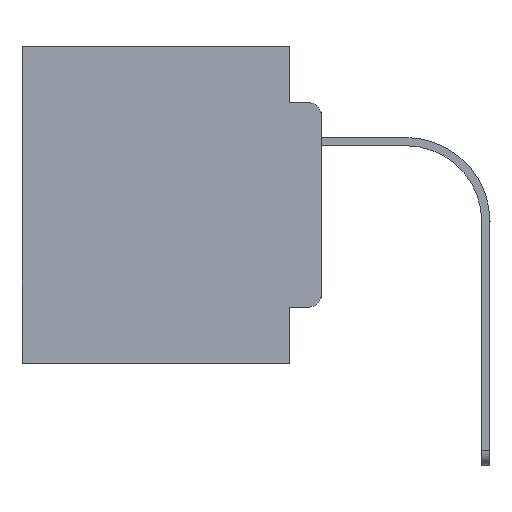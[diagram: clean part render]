
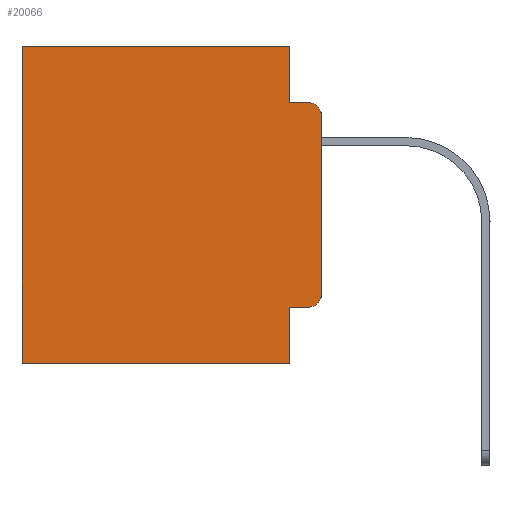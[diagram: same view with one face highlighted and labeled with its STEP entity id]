
A CAD part, left-side view. The second image highlights one B-rep face of the part: STEP entity #20066.
In plain terms, the highlighted planar face has unit normal (-1, 0, 0).
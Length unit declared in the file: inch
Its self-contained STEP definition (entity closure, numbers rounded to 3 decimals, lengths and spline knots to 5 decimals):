
#27 = LINE ( 'NONE', #24233, #23879 ) ;
#28 = DIRECTION ( 'NONE',  ( -1., 0., 0. ) ) ;
#840 = CARTESIAN_POINT ( 'NONE',  ( 0.298, 0.473, 0. ) ) ;
#1230 = ORIENTED_EDGE ( 'NONE', *, *, #2254, .F. ) ;
#1578 = CIRCLE ( 'NONE', #19807, 0.02 ) ;
#1582 = VECTOR ( 'NONE', #14883, 39.37008 ) ;
#1724 = FACE_OUTER_BOUND ( 'NONE', #25973, .T. ) ;
#2254 = EDGE_CURVE ( 'NONE', #10997, #7999, #5723, .T. ) ;
#2486 = EDGE_CURVE ( 'NONE', #16916, #17558, #19081, .T. ) ;
#2746 = CARTESIAN_POINT ( 'NONE',  ( 0.298, 0.02, -0.4115 ) ) ;
#3034 = DIRECTION ( 'NONE',  ( 0., 0., -1. ) ) ;
#3601 = DIRECTION ( 'NONE',  ( 0., 0., -1. ) ) ;
#3669 = EDGE_CURVE ( 'NONE', #10997, #20753, #16736, .T. ) ;
#3742 = CIRCLE ( 'NONE', #19013, 0.02 ) ;
#4521 = CARTESIAN_POINT ( 'NONE',  ( 0.298, 0.051, -0.4115 ) ) ;
#5129 = CARTESIAN_POINT ( 'NONE',  ( 0.298, 0.051, -0.0885 ) ) ;
#5399 = EDGE_CURVE ( 'NONE', #7165, #24015, #1578, .T. ) ;
#5652 = ORIENTED_EDGE ( 'NONE', *, *, #21985, .F. ) ;
#5718 = LINE ( 'NONE', #13822, #18164 ) ;
#5723 = LINE ( 'NONE', #19667, #22315 ) ;
#5754 = EDGE_CURVE ( 'NONE', #20785, #24015, #22165, .T. ) ;
#6103 = EDGE_CURVE ( 'NONE', #20753, #25151, #3742, .T. ) ;
#7036 = ORIENTED_EDGE ( 'NONE', *, *, #2486, .T. ) ;
#7165 = VERTEX_POINT ( 'NONE', #18683 ) ;
#7427 = ORIENTED_EDGE ( 'NONE', *, *, #5754, .F. ) ;
#7999 = VERTEX_POINT ( 'NONE', #25230 ) ;
#8914 = ORIENTED_EDGE ( 'NONE', *, *, #10478, .F. ) ;
#9082 = DIRECTION ( 'NONE',  ( 0., 1., 0. ) ) ;
#9113 = CARTESIAN_POINT ( 'NONE',  ( 0.298, 0., -0.3915 ) ) ;
#9138 = DIRECTION ( 'NONE',  ( 0., 0., -1. ) ) ;
#9844 = DIRECTION ( 'NONE',  ( 0., 1., 0. ) ) ;
#10046 = ORIENTED_EDGE ( 'NONE', *, *, #5399, .T. ) ;
#10109 = CARTESIAN_POINT ( 'NONE',  ( 0.298, 0., 0. ) ) ;
#10478 = EDGE_CURVE ( 'NONE', #7165, #25151, #27, .T. ) ;
#10844 = EDGE_CURVE ( 'NONE', #7999, #17558, #5718, .T. ) ;
#10997 = VERTEX_POINT ( 'NONE', #16455 ) ;
#11525 = DIRECTION ( 'NONE',  ( 0., 0., -1. ) ) ;
#12053 = EDGE_CURVE ( 'NONE', #13106, #16916, #17548, .T. ) ;
#12131 = DIRECTION ( 'NONE',  ( 0., 0., -1. ) ) ;
#12497 = DIRECTION ( 'NONE',  ( 0., 0., -1. ) ) ;
#13106 = VERTEX_POINT ( 'NONE', #16250 ) ;
#13734 = ORIENTED_EDGE ( 'NONE', *, *, #12053, .T. ) ;
#13822 = CARTESIAN_POINT ( 'NONE',  ( 0.298, 0., -0.5 ) ) ;
#14144 = VECTOR ( 'NONE', #9138, 39.37008 ) ;
#14503 = CARTESIAN_POINT ( 'NONE',  ( 0.298, 0.02, -0.3915 ) ) ;
#14596 = CARTESIAN_POINT ( 'NONE',  ( 0.298, 0.02, -0.1085 ) ) ;
#14816 = VECTOR ( 'NONE', #9082, 39.37008 ) ;
#14883 = DIRECTION ( 'NONE',  ( 0., -1., 0. ) ) ;
#15540 = VECTOR ( 'NONE', #11525, 39.37008 ) ;
#16214 = CARTESIAN_POINT ( 'NONE',  ( 0.298, 0.02, -0.0885 ) ) ;
#16250 = CARTESIAN_POINT ( 'NONE',  ( 0.298, 0.051, 0. ) ) ;
#16455 = CARTESIAN_POINT ( 'NONE',  ( 0.298, 0.051, -0.4115 ) ) ;
#16736 = LINE ( 'NONE', #4521, #1582 ) ;
#16776 = ORIENTED_EDGE ( 'NONE', *, *, #3669, .T. ) ;
#16916 = VERTEX_POINT ( 'NONE', #840 ) ;
#16955 = LINE ( 'NONE', #21750, #14144 ) ;
#17548 = LINE ( 'NONE', #19153, #14816 ) ;
#17558 = VERTEX_POINT ( 'NONE', #25674 ) ;
#18160 = CARTESIAN_POINT ( 'NONE',  ( 0.298, 0.051, -0.0885 ) ) ;
#18164 = VECTOR ( 'NONE', #9844, 39.37008 ) ;
#18340 = PLANE ( 'NONE',  #26035 ) ;
#18683 = CARTESIAN_POINT ( 'NONE',  ( 0.298, 0., -0.1085 ) ) ;
#18747 = DIRECTION ( 'NONE',  ( 0., 0., -1. ) ) ;
#19013 = AXIS2_PLACEMENT_3D ( 'NONE', #14503, #28, #18747 ) ;
#19081 = LINE ( 'NONE', #19211, #15540 ) ;
#19153 = CARTESIAN_POINT ( 'NONE',  ( 0.298, 0., 0. ) ) ;
#19211 = CARTESIAN_POINT ( 'NONE',  ( 0.298, 0.473, 0. ) ) ;
#19667 = CARTESIAN_POINT ( 'NONE',  ( 0.298, 0.051, 0. ) ) ;
#19807 = AXIS2_PLACEMENT_3D ( 'NONE', #14596, #24842, #3034 ) ;
#20066 = ADVANCED_FACE ( 'NONE', ( #1724 ), #18340, .F. ) ;
#20753 = VERTEX_POINT ( 'NONE', #2746 ) ;
#20785 = VERTEX_POINT ( 'NONE', #5129 ) ;
#21564 = ORIENTED_EDGE ( 'NONE', *, *, #10844, .F. ) ;
#21750 = CARTESIAN_POINT ( 'NONE',  ( 0.298, 0.051, 0. ) ) ;
#21985 = EDGE_CURVE ( 'NONE', #13106, #20785, #16955, .T. ) ;
#22165 = LINE ( 'NONE', #18160, #23264 ) ;
#22315 = VECTOR ( 'NONE', #3601, 39.37008 ) ;
#23264 = VECTOR ( 'NONE', #24561, 39.37008 ) ;
#23879 = VECTOR ( 'NONE', #12131, 39.37008 ) ;
#24015 = VERTEX_POINT ( 'NONE', #16214 ) ;
#24211 = DIRECTION ( 'NONE',  ( 1., 0., 0. ) ) ;
#24233 = CARTESIAN_POINT ( 'NONE',  ( 0.298, 0., 0. ) ) ;
#24561 = DIRECTION ( 'NONE',  ( 0., -1., 0. ) ) ;
#24842 = DIRECTION ( 'NONE',  ( -1., 0., 0. ) ) ;
#25151 = VERTEX_POINT ( 'NONE', #9113 ) ;
#25230 = CARTESIAN_POINT ( 'NONE',  ( 0.298, 0.051, -0.5 ) ) ;
#25674 = CARTESIAN_POINT ( 'NONE',  ( 0.298, 0.473, -0.5 ) ) ;
#25836 = ORIENTED_EDGE ( 'NONE', *, *, #6103, .T. ) ;
#25973 = EDGE_LOOP ( 'NONE', ( #8914, #10046, #7427, #5652, #13734, #7036, #21564, #1230, #16776, #25836 ) ) ;
#26035 = AXIS2_PLACEMENT_3D ( 'NONE', #10109, #24211, #12497 ) ;
